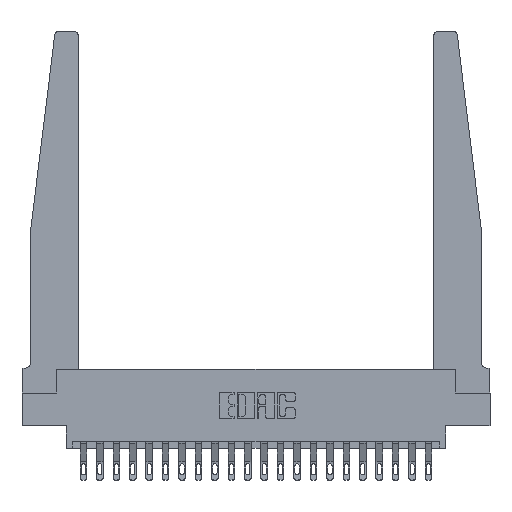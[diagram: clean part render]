
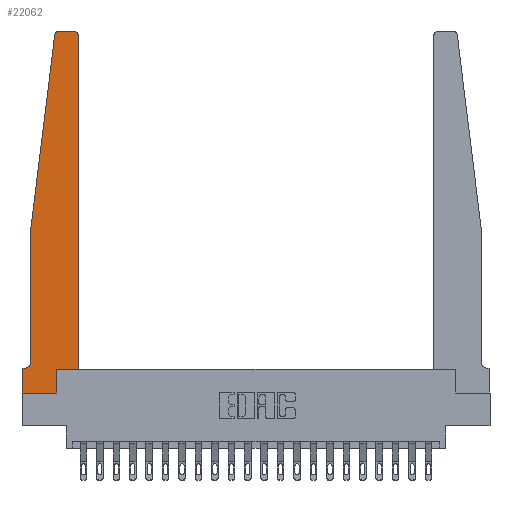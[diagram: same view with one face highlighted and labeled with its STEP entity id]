
A CAD part, top view. The second image highlights one B-rep face of the part: STEP entity #22062.
In plain terms, the highlighted planar face has unit normal (0, 0, 1).
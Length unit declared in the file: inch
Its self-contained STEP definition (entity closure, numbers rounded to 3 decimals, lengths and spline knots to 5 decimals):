
#465 = VECTOR ( 'NONE', #20044, 39.37008 ) ;
#510 = DIRECTION ( 'NONE',  ( 0., -1., 0. ) ) ;
#553 = EDGE_CURVE ( 'NONE', #1421, #12239, #18356, .T. ) ;
#726 = DIRECTION ( 'NONE',  ( 0., 0., 1. ) ) ;
#1042 = CARTESIAN_POINT ( 'NONE',  ( 0.015, 0.1875, 0.37 ) ) ;
#1068 = EDGE_CURVE ( 'NONE', #15279, #9349, #8992, .T. ) ;
#1179 = VECTOR ( 'NONE', #9038, 39.37008 ) ;
#1421 = VERTEX_POINT ( 'NONE', #6609 ) ;
#1580 = EDGE_CURVE ( 'NONE', #14134, #15279, #22072, .T. ) ;
#1678 = AXIS2_PLACEMENT_3D ( 'NONE', #11119, #726, #12825 ) ;
#2214 = ORIENTED_EDGE ( 'NONE', *, *, #15906, .T. ) ;
#2754 = ORIENTED_EDGE ( 'NONE', *, *, #7051, .T. ) ;
#3012 = DIRECTION ( 'NONE',  ( 0., 0., -1. ) ) ;
#3707 = ORIENTED_EDGE ( 'NONE', *, *, #21412, .T. ) ;
#4084 = DIRECTION ( 'NONE',  ( -1., 0., 0. ) ) ;
#4214 = EDGE_LOOP ( 'NONE', ( #2754, #13474, #6651, #15217, #2214, #6499, #15865, #11532, #13590, #17347, #3707, #9420 ) ) ;
#4317 = VERTEX_POINT ( 'NONE', #9618 ) ;
#4489 = CARTESIAN_POINT ( 'NONE',  ( 0., 0., 0.37 ) ) ;
#4798 = VERTEX_POINT ( 'NONE', #8838 ) ;
#5431 = VERTEX_POINT ( 'NONE', #5782 ) ;
#5477 = LINE ( 'NONE', #14387, #15162 ) ;
#5585 = VERTEX_POINT ( 'NONE', #13075 ) ;
#5782 = CARTESIAN_POINT ( 'NONE',  ( 0.24675, 2.72367, 0.37 ) ) ;
#6294 = EDGE_CURVE ( 'NONE', #9349, #15196, #10393, .T. ) ;
#6499 = ORIENTED_EDGE ( 'NONE', *, *, #1580, .T. ) ;
#6609 = CARTESIAN_POINT ( 'NONE',  ( 0.2605, 0.18, 0.37 ) ) ;
#6651 = ORIENTED_EDGE ( 'NONE', *, *, #15190, .T. ) ;
#6663 = LINE ( 'NONE', #20165, #19797 ) ;
#6768 = VERTEX_POINT ( 'NONE', #13578 ) ;
#6876 = EDGE_CURVE ( 'NONE', #6768, #5431, #8740, .T. ) ;
#7051 = EDGE_CURVE ( 'NONE', #5585, #6768, #5477, .T. ) ;
#7152 = DIRECTION ( 'NONE',  ( 0., 0., 1. ) ) ;
#7267 = AXIS2_PLACEMENT_3D ( 'NONE', #13353, #3012, #15070 ) ;
#8740 = CIRCLE ( 'NONE', #21061, 0.03 ) ;
#8838 = CARTESIAN_POINT ( 'NONE',  ( 0.065, 1.25, 0.37 ) ) ;
#8974 = VECTOR ( 'NONE', #13846, 39.37008 ) ;
#8992 = LINE ( 'NONE', #14316, #18095 ) ;
#9038 = DIRECTION ( 'NONE',  ( 1., 0., 0. ) ) ;
#9132 = CARTESIAN_POINT ( 'NONE',  ( 0.065, 1.25, 0.37 ) ) ;
#9349 = VERTEX_POINT ( 'NONE', #4489 ) ;
#9420 = ORIENTED_EDGE ( 'NONE', *, *, #14066, .T. ) ;
#9618 = CARTESIAN_POINT ( 'NONE',  ( 0.065, 0.2375, 0.37 ) ) ;
#9894 = CARTESIAN_POINT ( 'NONE',  ( 0., 0.1875, 0.37 ) ) ;
#10393 = LINE ( 'NONE', #12420, #1179 ) ;
#10427 = VECTOR ( 'NONE', #15915, 39.37008 ) ;
#10784 = CARTESIAN_POINT ( 'NONE',  ( 0.2605, 0.18, 0.37 ) ) ;
#11054 = EDGE_CURVE ( 'NONE', #15196, #1421, #19531, .T. ) ;
#11117 = CARTESIAN_POINT ( 'NONE',  ( 0.425, 0.18, 0.37 ) ) ;
#11119 = CARTESIAN_POINT ( 'NONE',  ( 0.395, 2.72, 0.37 ) ) ;
#11380 = VECTOR ( 'NONE', #17160, 39.37008 ) ;
#11526 = CARTESIAN_POINT ( 'NONE',  ( 0.425, 0.18, 0.37 ) ) ;
#11532 = ORIENTED_EDGE ( 'NONE', *, *, #6294, .T. ) ;
#11624 = DIRECTION ( 'NONE',  ( 1., 0., 0. ) ) ;
#11660 = LINE ( 'NONE', #9132, #20220 ) ;
#12239 = VERTEX_POINT ( 'NONE', #11117 ) ;
#12420 = CARTESIAN_POINT ( 'NONE',  ( 0., 0., 0.37 ) ) ;
#12524 = FACE_OUTER_BOUND ( 'NONE', #4214, .T. ) ;
#12586 = DIRECTION ( 'NONE',  ( -0.122, -0.992, 0. ) ) ;
#12804 = CARTESIAN_POINT ( 'NONE',  ( 0., 0.1875, 0.37 ) ) ;
#12825 = DIRECTION ( 'NONE',  ( 1., 0., 0. ) ) ;
#13075 = CARTESIAN_POINT ( 'NONE',  ( 0.395, 2.75, 0.37 ) ) ;
#13254 = PLANE ( 'NONE',  #20132 ) ;
#13353 = CARTESIAN_POINT ( 'NONE',  ( 0.015, 0.2375, 0.37 ) ) ;
#13474 = ORIENTED_EDGE ( 'NONE', *, *, #6876, .T. ) ;
#13578 = CARTESIAN_POINT ( 'NONE',  ( 0.27653, 2.75, 0.37 ) ) ;
#13590 = ORIENTED_EDGE ( 'NONE', *, *, #11054, .T. ) ;
#13718 = CARTESIAN_POINT ( 'NONE',  ( 0.065, 1.25, 0.37 ) ) ;
#13801 = EDGE_CURVE ( 'NONE', #4798, #4317, #16974, .T. ) ;
#13846 = DIRECTION ( 'NONE',  ( -1., 0., 0. ) ) ;
#14066 = EDGE_CURVE ( 'NONE', #17925, #5585, #21320, .T. ) ;
#14134 = VERTEX_POINT ( 'NONE', #1042 ) ;
#14316 = CARTESIAN_POINT ( 'NONE',  ( 0., 0., 0.37 ) ) ;
#14387 = CARTESIAN_POINT ( 'NONE',  ( 0.25, 2.75, 0.37 ) ) ;
#14935 = CARTESIAN_POINT ( 'NONE',  ( 0.425, 2.72, 0.37 ) ) ;
#15070 = DIRECTION ( 'NONE',  ( -1., 0., 0. ) ) ;
#15162 = VECTOR ( 'NONE', #4084, 39.37008 ) ;
#15190 = EDGE_CURVE ( 'NONE', #5431, #4798, #11660, .T. ) ;
#15196 = VERTEX_POINT ( 'NONE', #16005 ) ;
#15217 = ORIENTED_EDGE ( 'NONE', *, *, #13801, .T. ) ;
#15279 = VERTEX_POINT ( 'NONE', #12804 ) ;
#15865 = ORIENTED_EDGE ( 'NONE', *, *, #1068, .T. ) ;
#15906 = EDGE_CURVE ( 'NONE', #4317, #14134, #20974, .T. ) ;
#15915 = DIRECTION ( 'NONE',  ( 0., 1., 0. ) ) ;
#16005 = CARTESIAN_POINT ( 'NONE',  ( 0.2605, 0., 0.37 ) ) ;
#16974 = LINE ( 'NONE', #13718, #11380 ) ;
#17160 = DIRECTION ( 'NONE',  ( 0., -1., 0. ) ) ;
#17293 = CARTESIAN_POINT ( 'NONE',  ( 0.065, 0.1875, 0.37 ) ) ;
#17347 = ORIENTED_EDGE ( 'NONE', *, *, #553, .T. ) ;
#17387 = CARTESIAN_POINT ( 'NONE',  ( 0.27653, 2.72, 0.37 ) ) ;
#17925 = VERTEX_POINT ( 'NONE', #14935 ) ;
#18095 = VECTOR ( 'NONE', #510, 39.37008 ) ;
#18356 = LINE ( 'NONE', #11526, #465 ) ;
#18439 = DIRECTION ( 'NONE',  ( 0., 1., 0. ) ) ;
#19128 = DIRECTION ( 'NONE',  ( 1., 0., 0. ) ) ;
#19531 = LINE ( 'NONE', #10784, #10427 ) ;
#19797 = VECTOR ( 'NONE', #18439, 39.37008 ) ;
#20044 = DIRECTION ( 'NONE',  ( 1., 0., 0. ) ) ;
#20132 = AXIS2_PLACEMENT_3D ( 'NONE', #9894, #21845, #11624 ) ;
#20165 = CARTESIAN_POINT ( 'NONE',  ( 0.425, 0.18, 0.37 ) ) ;
#20220 = VECTOR ( 'NONE', #12586, 39.37008 ) ;
#20974 = CIRCLE ( 'NONE', #7267, 0.05 ) ;
#21061 = AXIS2_PLACEMENT_3D ( 'NONE', #17387, #7152, #19128 ) ;
#21320 = CIRCLE ( 'NONE', #1678, 0.03 ) ;
#21412 = EDGE_CURVE ( 'NONE', #12239, #17925, #6663, .T. ) ;
#21845 = DIRECTION ( 'NONE',  ( 0., 0., 1. ) ) ;
#22062 = ADVANCED_FACE ( 'NONE', ( #12524 ), #13254, .T. ) ;
#22072 = LINE ( 'NONE', #17293, #8974 ) ;
